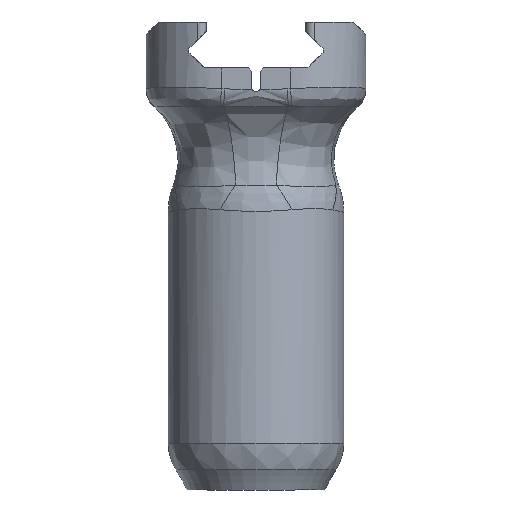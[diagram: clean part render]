
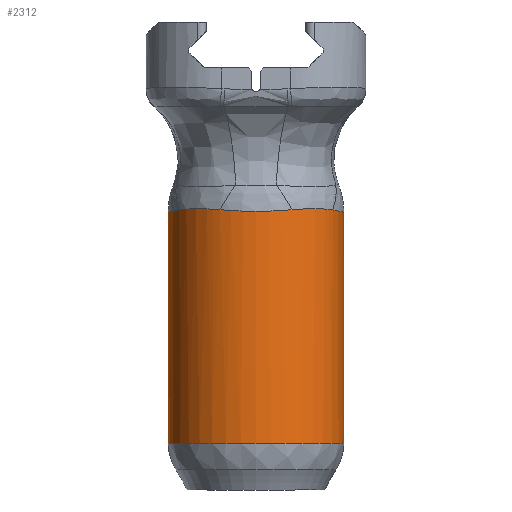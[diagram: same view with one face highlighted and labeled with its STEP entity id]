
A CAD part, front view. The second image highlights one B-rep face of the part: STEP entity #2312.
In plain terms, the highlighted cylindrical face has radius 14 mm (diameter 28 mm), a partial arc.
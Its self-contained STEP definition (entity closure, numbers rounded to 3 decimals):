
#133=B_SPLINE_CURVE_WITH_KNOTS('',3,(#4633,#4634,#4635,#4636,#4637),
 .UNSPECIFIED.,.F.,.F.,(4,1,4),(0.,0.047,0.11),
 .UNSPECIFIED.);
#134=B_SPLINE_CURVE_WITH_KNOTS('',3,(#4639,#4640,#4641,#4642,#4643,#4644,
#4645,#4646,#4647,#4648,#4649,#4650,#4651),.UNSPECIFIED.,.F.,.F.,(4,1,1,
1,1,1,1,1,1,1,4),(0.,0.01,0.019,0.038,
0.058,0.077,0.096,0.115,
0.125,0.129,0.134),.UNSPECIFIED.);
#135=B_SPLINE_CURVE_WITH_KNOTS('',3,(#4653,#4654,#4655,#4656,#4657,#4658,
#4659),.UNSPECIFIED.,.F.,.F.,(4,1,1,1,4),(0.,0.051,0.077,
0.128,0.179),.UNSPECIFIED.);
#136=B_SPLINE_CURVE_WITH_KNOTS('',3,(#4661,#4662,#4663,#4664,#4665,#4666,
#4667,#4668,#4669,#4670,#4671),.UNSPECIFIED.,.F.,.F.,(4,1,1,1,1,1,1,1,4),
(0.,0.005,0.01,0.019,
0.038,0.077,0.115,0.125,
0.134),.UNSPECIFIED.);
#137=B_SPLINE_CURVE_WITH_KNOTS('',3,(#4672,#4673,#4674,#4675,#4676),
 .UNSPECIFIED.,.F.,.F.,(4,1,4),(0.,0.047,0.11),
 .UNSPECIFIED.);
#236=LINE('',#3387,#371);
#244=LINE('',#3450,#379);
#371=VECTOR('',#2786,10.);
#379=VECTOR('',#2826,10.);
#506=CYLINDRICAL_SURFACE('',#2573,14.);
#631=FACE_OUTER_BOUND('',#774,.T.);
#774=EDGE_LOOP('',(#2088,#2089,#2090,#2091,#2092,#2093,#2094,#2095));
#841=CIRCLE('',#2430,14.);
#957=VERTEX_POINT('',#3383);
#959=VERTEX_POINT('',#3386);
#965=VERTEX_POINT('',#3432);
#968=VERTEX_POINT('',#3447);
#1114=VERTEX_POINT('',#4632);
#1115=VERTEX_POINT('',#4638);
#1116=VERTEX_POINT('',#4652);
#1117=VERTEX_POINT('',#4660);
#1202=EDGE_CURVE('',#959,#957,#236,.T.);
#1211=EDGE_CURVE('',#959,#965,#841,.T.);
#1221=EDGE_CURVE('',#965,#968,#244,.T.);
#1445=EDGE_CURVE('',#1114,#957,#133,.T.);
#1446=EDGE_CURVE('',#1115,#1114,#134,.T.);
#1447=EDGE_CURVE('',#1116,#1115,#135,.T.);
#1448=EDGE_CURVE('',#1117,#1116,#136,.T.);
#1449=EDGE_CURVE('',#968,#1117,#137,.T.);
#2088=ORIENTED_EDGE('',*,*,#1445,.F.);
#2089=ORIENTED_EDGE('',*,*,#1446,.F.);
#2090=ORIENTED_EDGE('',*,*,#1447,.F.);
#2091=ORIENTED_EDGE('',*,*,#1448,.F.);
#2092=ORIENTED_EDGE('',*,*,#1449,.F.);
#2093=ORIENTED_EDGE('',*,*,#1221,.F.);
#2094=ORIENTED_EDGE('',*,*,#1211,.F.);
#2095=ORIENTED_EDGE('',*,*,#1202,.T.);
#2312=ADVANCED_FACE('',(#631),#506,.T.);
#2430=AXIS2_PLACEMENT_3D('',#3433,#2802,#2803);
#2573=AXIS2_PLACEMENT_3D('',#4631,#3185,#3186);
#2786=DIRECTION('',(0.,0.,1.));
#2802=DIRECTION('center_axis',(0.,0.,
-1.));
#2803=DIRECTION('ref_axis',(0.,-1.,0.));
#2826=DIRECTION('',(0.,0.,1.));
#3185=DIRECTION('center_axis',(0.,0.,
1.));
#3186=DIRECTION('ref_axis',(1.,0.,0.));
#3383=CARTESIAN_POINT('',(14.,50.504,83.476));
#3386=CARTESIAN_POINT('',(14.,50.504,46.681));
#3387=CARTESIAN_POINT('',(14.,50.504,39.193));
#3432=CARTESIAN_POINT('',(-14.,50.504,46.681));
#3433=CARTESIAN_POINT('Origin',(0.,50.504,46.681));
#3447=CARTESIAN_POINT('',(-14.,50.504,83.476));
#3450=CARTESIAN_POINT('',(-14.,50.504,84.193));
#4631=CARTESIAN_POINT('Origin',(0.,50.504,39.193));
#4632=CARTESIAN_POINT('',(12.235,43.699,83.848));
#4633=CARTESIAN_POINT('Ctrl Pts',(12.235,43.699,83.848));
#4634=CARTESIAN_POINT('Ctrl Pts',(12.665,44.472,83.754));
#4635=CARTESIAN_POINT('Ctrl Pts',(13.573,46.496,83.562));
#4636=CARTESIAN_POINT('Ctrl Pts',(14.,49.037,83.476));
#4637=CARTESIAN_POINT('Ctrl Pts',(14.,50.504,83.476));
#4638=CARTESIAN_POINT('',(5.752,37.74,83.884));
#4639=CARTESIAN_POINT('Ctrl Pts',(5.752,37.74,83.884));
#4640=CARTESIAN_POINT('Ctrl Pts',(5.927,37.819,83.9));
#4641=CARTESIAN_POINT('Ctrl Pts',(6.287,37.99,83.929));
#4642=CARTESIAN_POINT('Ctrl Pts',(7.022,38.379,83.977));
#4643=CARTESIAN_POINT('Ctrl Pts',(7.946,38.952,84.016));
#4644=CARTESIAN_POINT('Ctrl Pts',(9.012,39.762,84.037));
#4645=CARTESIAN_POINT('Ctrl Pts',(10.,40.675,84.033));
#4646=CARTESIAN_POINT('Ctrl Pts',(10.886,41.668,84.003));
#4647=CARTESIAN_POINT('Ctrl Pts',(11.521,42.531,83.955));
#4648=CARTESIAN_POINT('Ctrl Pts',(11.902,43.128,83.907));
#4649=CARTESIAN_POINT('Ctrl Pts',(12.1,43.46,83.875));
#4650=CARTESIAN_POINT('Ctrl Pts',(12.192,43.621,83.857));
#4651=CARTESIAN_POINT('Ctrl Pts',(12.235,43.699,83.848));
#4652=CARTESIAN_POINT('',(-5.752,37.74,83.884));
#4653=CARTESIAN_POINT('Ctrl Pts',(-5.752,37.74,83.884));
#4654=CARTESIAN_POINT('Ctrl Pts',(-4.818,37.319,83.796));
#4655=CARTESIAN_POINT('Ctrl Pts',(-3.243,36.798,83.69));
#4656=CARTESIAN_POINT('Ctrl Pts',(-0.313,36.416,83.613));
#4657=CARTESIAN_POINT('Ctrl Pts',(2.719,36.618,83.653));
#4658=CARTESIAN_POINT('Ctrl Pts',(4.818,37.319,83.796));
#4659=CARTESIAN_POINT('Ctrl Pts',(5.752,37.74,83.884));
#4660=CARTESIAN_POINT('',(-12.235,43.699,83.848));
#4661=CARTESIAN_POINT('Ctrl Pts',(-12.235,43.699,83.848));
#4662=CARTESIAN_POINT('Ctrl Pts',(-12.192,43.621,83.857));
#4663=CARTESIAN_POINT('Ctrl Pts',(-12.1,43.46,83.875));
#4664=CARTESIAN_POINT('Ctrl Pts',(-11.902,43.128,83.907));
#4665=CARTESIAN_POINT('Ctrl Pts',(-11.521,42.532,83.955));
#4666=CARTESIAN_POINT('Ctrl Pts',(-10.632,41.322,84.022));
#4667=CARTESIAN_POINT('Ctrl Pts',(-9.053,39.709,84.049));
#4668=CARTESIAN_POINT('Ctrl Pts',(-7.391,38.574,84.));
#4669=CARTESIAN_POINT('Ctrl Pts',(-6.286,37.99,83.929));
#4670=CARTESIAN_POINT('Ctrl Pts',(-5.927,37.819,83.9));
#4671=CARTESIAN_POINT('Ctrl Pts',(-5.752,37.74,83.884));
#4672=CARTESIAN_POINT('Ctrl Pts',(-14.,50.504,83.476));
#4673=CARTESIAN_POINT('Ctrl Pts',(-14.,49.404,83.476));
#4674=CARTESIAN_POINT('Ctrl Pts',(-13.683,46.843,83.54));
#4675=CARTESIAN_POINT('Ctrl Pts',(-12.808,44.729,83.723));
#4676=CARTESIAN_POINT('Ctrl Pts',(-12.235,43.699,83.848));
